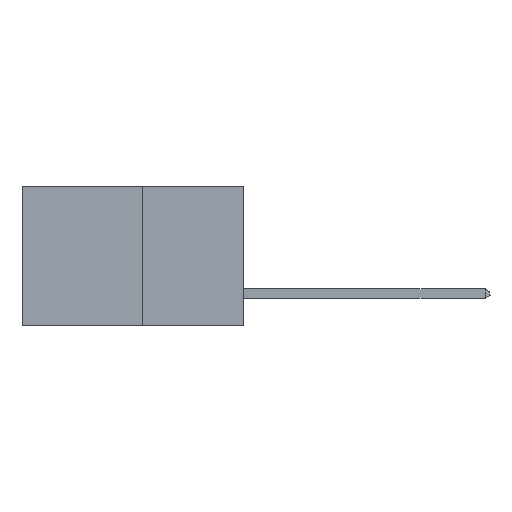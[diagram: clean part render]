
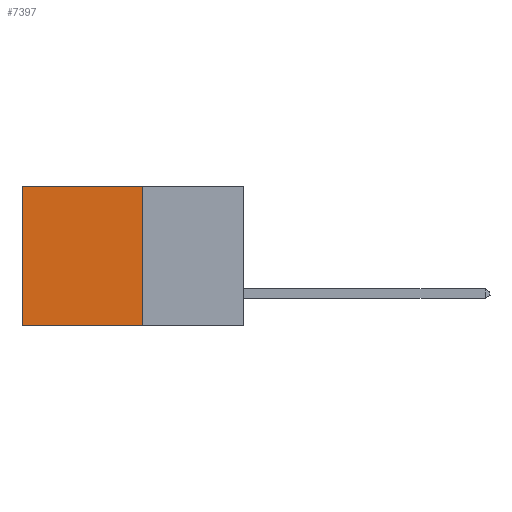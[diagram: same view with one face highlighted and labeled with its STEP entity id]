
A CAD part, left-side view. The second image highlights one B-rep face of the part: STEP entity #7397.
In plain terms, the highlighted planar face has unit normal (-1, 0, 0).
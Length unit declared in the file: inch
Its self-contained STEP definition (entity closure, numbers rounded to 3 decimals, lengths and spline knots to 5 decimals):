
#678 = CARTESIAN_POINT ( 'NONE',  ( 0.277, 0.59, -0.37 ) ) ;
#926 = EDGE_CURVE ( 'NONE', #14083, #8317, #13478, .T. ) ;
#1265 = DIRECTION ( 'NONE',  ( 0., 0., -1. ) ) ;
#3264 = VERTEX_POINT ( 'NONE', #3728 ) ;
#3728 = CARTESIAN_POINT ( 'NONE',  ( 0.277, 0.27, 0. ) ) ;
#4189 = DIRECTION ( 'NONE',  ( 0., 0., -1. ) ) ;
#4203 = CARTESIAN_POINT ( 'NONE',  ( 0.277, 0.27, -0.37 ) ) ;
#4251 = EDGE_CURVE ( 'NONE', #3264, #11373, #15279, .T. ) ;
#5100 = CARTESIAN_POINT ( 'NONE',  ( 0.277, 0.27, -0.37 ) ) ;
#5127 = VECTOR ( 'NONE', #11950, 39.37008 ) ;
#5704 = CARTESIAN_POINT ( 'NONE',  ( 0.277, 0.27, -0.37 ) ) ;
#5871 = EDGE_LOOP ( 'NONE', ( #12634, #6610, #14651, #15405 ) ) ;
#5891 = LINE ( 'NONE', #4203, #14906 ) ;
#6132 = FACE_OUTER_BOUND ( 'NONE', #5871, .T. ) ;
#6481 = CARTESIAN_POINT ( 'NONE',  ( 0.277, 0.59, -0.37 ) ) ;
#6610 = ORIENTED_EDGE ( 'NONE', *, *, #926, .F. ) ;
#7273 = DIRECTION ( 'NONE',  ( 0., 1., 0. ) ) ;
#7397 = ADVANCED_FACE ( 'NONE', ( #6132 ), #12030, .F. ) ;
#7651 = EDGE_CURVE ( 'NONE', #11373, #8317, #11659, .T. ) ;
#8317 = VERTEX_POINT ( 'NONE', #6481 ) ;
#8504 = EDGE_CURVE ( 'NONE', #3264, #14083, #5891, .T. ) ;
#9226 = CARTESIAN_POINT ( 'NONE',  ( 0.277, 0.59, 0. ) ) ;
#9705 = CARTESIAN_POINT ( 'NONE',  ( 0.277, 0.27, 0. ) ) ;
#10524 = DIRECTION ( 'NONE',  ( 0., 0., -1. ) ) ;
#10559 = DIRECTION ( 'NONE',  ( 1., 0., 0. ) ) ;
#10812 = CARTESIAN_POINT ( 'NONE',  ( 0.277, 0.27, -0.37 ) ) ;
#11373 = VERTEX_POINT ( 'NONE', #9226 ) ;
#11659 = LINE ( 'NONE', #678, #14933 ) ;
#11950 = DIRECTION ( 'NONE',  ( 0., 1., 0. ) ) ;
#12030 = PLANE ( 'NONE',  #12263 ) ;
#12263 = AXIS2_PLACEMENT_3D ( 'NONE', #10812, #10559, #10524 ) ;
#12313 = VECTOR ( 'NONE', #7273, 39.37008 ) ;
#12634 = ORIENTED_EDGE ( 'NONE', *, *, #7651, .T. ) ;
#13478 = LINE ( 'NONE', #5704, #12313 ) ;
#14083 = VERTEX_POINT ( 'NONE', #5100 ) ;
#14651 = ORIENTED_EDGE ( 'NONE', *, *, #8504, .F. ) ;
#14906 = VECTOR ( 'NONE', #4189, 39.37008 ) ;
#14933 = VECTOR ( 'NONE', #1265, 39.37008 ) ;
#15279 = LINE ( 'NONE', #9705, #5127 ) ;
#15405 = ORIENTED_EDGE ( 'NONE', *, *, #4251, .T. ) ;
